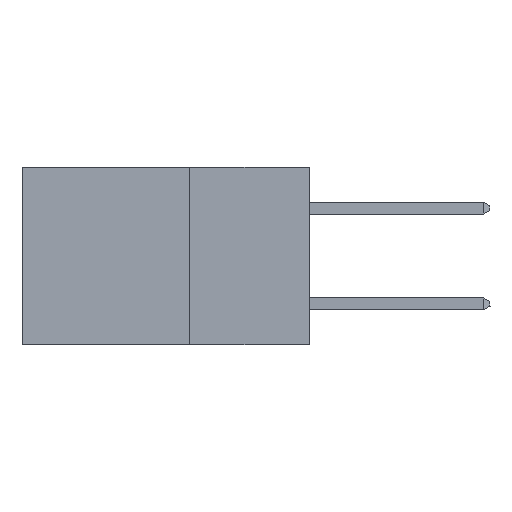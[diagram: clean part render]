
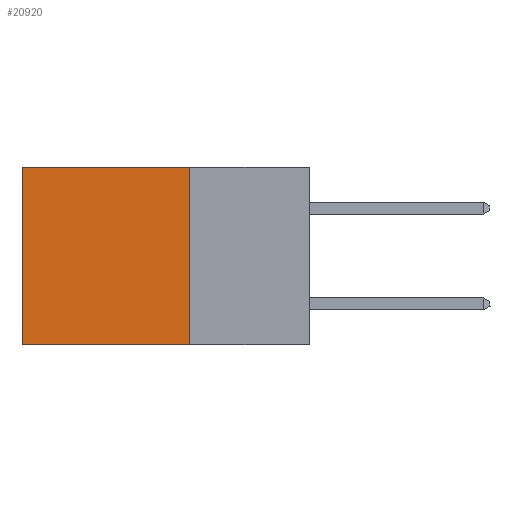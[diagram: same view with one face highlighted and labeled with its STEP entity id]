
A CAD part, left-side view. The second image highlights one B-rep face of the part: STEP entity #20920.
In plain terms, the highlighted planar face has unit normal (-1, 0, 0).
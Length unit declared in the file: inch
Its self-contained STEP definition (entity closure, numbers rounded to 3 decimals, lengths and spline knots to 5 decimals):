
#242 = DIRECTION ( 'NONE',  ( 0., 1., 0. ) ) ;
#417 = EDGE_CURVE ( 'NONE', #7753, #14593, #15053, .T. ) ;
#1160 = VECTOR ( 'NONE', #4563, 39.37008 ) ;
#1374 = ORIENTED_EDGE ( 'NONE', *, *, #14889, .F. ) ;
#1947 = LINE ( 'NONE', #10553, #3794 ) ;
#2407 = DIRECTION ( 'NONE',  ( 0., 0., -1. ) ) ;
#3506 = CARTESIAN_POINT ( 'NONE',  ( 0.2875, 0.25, -0.37 ) ) ;
#3794 = VECTOR ( 'NONE', #14288, 39.37008 ) ;
#4563 = DIRECTION ( 'NONE',  ( 0., 1., 0. ) ) ;
#5164 = VERTEX_POINT ( 'NONE', #6791 ) ;
#6791 = CARTESIAN_POINT ( 'NONE',  ( 0.2875, 0.25, 0. ) ) ;
#6919 = CARTESIAN_POINT ( 'NONE',  ( 0.2875, 0.6, -0.37 ) ) ;
#7678 = AXIS2_PLACEMENT_3D ( 'NONE', #16945, #21053, #17308 ) ;
#7753 = VERTEX_POINT ( 'NONE', #10785 ) ;
#8337 = FACE_OUTER_BOUND ( 'NONE', #16625, .T. ) ;
#8507 = VECTOR ( 'NONE', #242, 39.37008 ) ;
#8635 = VECTOR ( 'NONE', #2407, 39.37008 ) ;
#10310 = VERTEX_POINT ( 'NONE', #3506 ) ;
#10553 = CARTESIAN_POINT ( 'NONE',  ( 0.2875, 0.25, 0. ) ) ;
#10785 = CARTESIAN_POINT ( 'NONE',  ( 0.2875, 0.6, 0. ) ) ;
#12262 = CARTESIAN_POINT ( 'NONE',  ( 0.2875, 0.6, 0. ) ) ;
#13187 = ORIENTED_EDGE ( 'NONE', *, *, #17687, .F. ) ;
#14288 = DIRECTION ( 'NONE',  ( 0., 0., -1. ) ) ;
#14292 = LINE ( 'NONE', #23698, #8507 ) ;
#14593 = VERTEX_POINT ( 'NONE', #6919 ) ;
#14889 = EDGE_CURVE ( 'NONE', #10310, #14593, #14292, .T. ) ;
#15053 = LINE ( 'NONE', #12262, #8635 ) ;
#16257 = CARTESIAN_POINT ( 'NONE',  ( 0.2875, 0.25, 0. ) ) ;
#16401 = ORIENTED_EDGE ( 'NONE', *, *, #23278, .T. ) ;
#16625 = EDGE_LOOP ( 'NONE', ( #21644, #1374, #13187, #16401 ) ) ;
#16945 = CARTESIAN_POINT ( 'NONE',  ( 0.2875, 0.25, 0. ) ) ;
#17308 = DIRECTION ( 'NONE',  ( 0., 0., -1. ) ) ;
#17687 = EDGE_CURVE ( 'NONE', #5164, #10310, #1947, .T. ) ;
#17991 = LINE ( 'NONE', #16257, #1160 ) ;
#20920 = ADVANCED_FACE ( 'NONE', ( #8337 ), #24715, .F. ) ;
#21053 = DIRECTION ( 'NONE',  ( 1., 0., 0. ) ) ;
#21644 = ORIENTED_EDGE ( 'NONE', *, *, #417, .T. ) ;
#23278 = EDGE_CURVE ( 'NONE', #5164, #7753, #17991, .T. ) ;
#23698 = CARTESIAN_POINT ( 'NONE',  ( 0.2875, 0.25, -0.37 ) ) ;
#24715 = PLANE ( 'NONE',  #7678 ) ;
